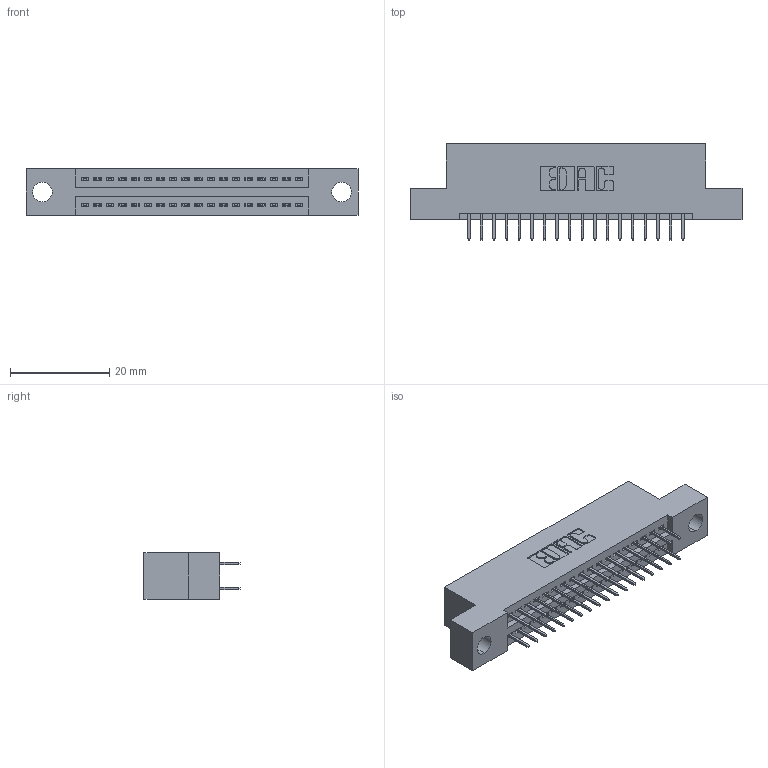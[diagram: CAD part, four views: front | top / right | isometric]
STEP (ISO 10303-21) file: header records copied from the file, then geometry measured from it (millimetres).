
FILE_DESCRIPTION (( 'STEP AP203' ), '1' );
FILE_NAME ('345-036-524-204.STEP', '2021-05-20T00:22:41', ( '' ), ( '' ), 'SwSTEP 2.0', 'SolidWorks 2020', '' );
FILE_SCHEMA (( 'CONFIG_CONTROL_DESIGN' ));
Length unit declared in the file: inch
Products named in the file (3): 345 Part_Flush Mounting Lugs - 0.156 Dia-TI; 345-036-524-204; 345-292-001_345-293-124
Assembly tree (37 placements, depth 2):
  345-036-524-204
    345 Part_Flush Mounting Lugs - 0.156 Dia-TI
    345-292-001_345-293-124  x36
Bounding box: 66.93 x 19.35 x 9.4 mm (x, y, z)
Volume: 6118.3 mm3; surface area: 8286.9 mm2
Topology: 37 solids, 37 shells, 2084 faces, 5885 edges, 3778 vertices
Faces by surface type: plane 1498, cylinder 586
Entity records: 17847 total; most frequent: CARTESIAN_POINT 3018, ORIENTED_EDGE 2950, DIRECTION 2691, EDGE_CURVE 1475, LINE 1275, VECTOR 1275, VERTEX_POINT 978, AXIS2_PLACEMENT_3D 708
